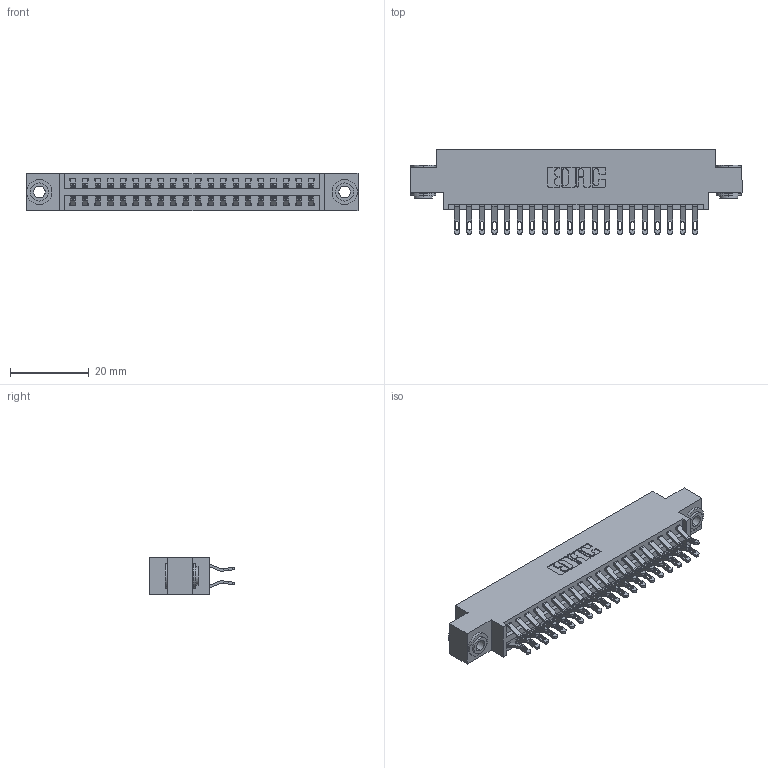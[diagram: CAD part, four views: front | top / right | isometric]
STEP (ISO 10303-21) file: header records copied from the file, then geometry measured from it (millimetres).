
FILE_DESCRIPTION (( 'STEP AP203' ), '1' );
FILE_NAME ('396-040-555-803.STEP', '2019-11-02T05:51:13', ( '' ), ( '' ), 'SwSTEP 2.0', 'SolidWorks 2016', '' );
FILE_SCHEMA (( 'CONFIG_CONTROL_DESIGN' ));
Length unit declared in the file: inch
Products named in the file (4): 346 Part_0.170 Offset - 0.156 Dia-TH; 345-292-001_555 Tail; 345-250-002_345-250-002-102; 396-040-555-803
Assembly tree (43 placements, depth 2):
  396-040-555-803
    346 Part_0.170 Offset - 0.156 Dia-TH
    345-292-001_555 Tail  x40
    345-250-002_345-250-002-102  x2
Bounding box: 84.07 x 21.46 x 9.4 mm (x, y, z)
Volume: 8008.2 mm3; surface area: 11469.4 mm2
Topology: 43 solids, 43 shells, 2484 faces, 7737 edges, 5154 vertices
Faces by surface type: plane 1410, cylinder 1066, cone 8
Entity records: 17122 total; most frequent: CARTESIAN_POINT 2865, ORIENTED_EDGE 2762, DIRECTION 2575, EDGE_CURVE 1381, LINE 1125, VECTOR 1125, VERTEX_POINT 918, AXIS2_PLACEMENT_3D 725
